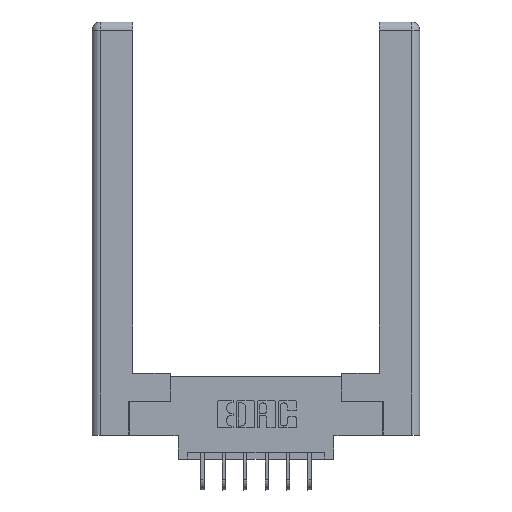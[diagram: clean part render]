
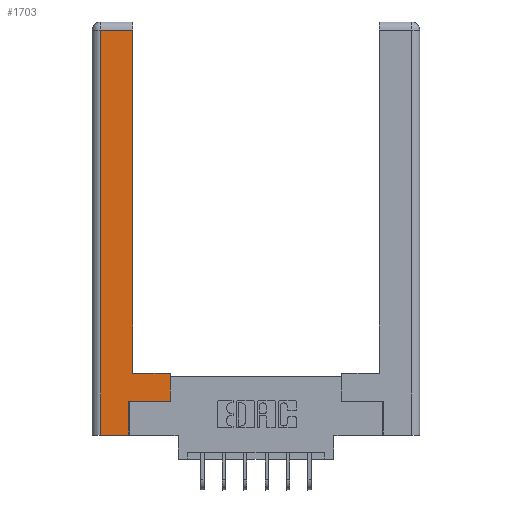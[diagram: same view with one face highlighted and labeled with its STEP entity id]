
A CAD part, top view. The second image highlights one B-rep face of the part: STEP entity #1703.
In plain terms, the highlighted planar face has unit normal (0, 0, 1).
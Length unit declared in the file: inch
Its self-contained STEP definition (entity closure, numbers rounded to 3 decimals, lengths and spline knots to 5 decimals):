
#116 = ORIENTED_EDGE ( 'NONE', *, *, #510, .T. ) ;
#121 = LINE ( 'NONE', #13574, #1933 ) ;
#510 = EDGE_CURVE ( 'NONE', #4263, #7107, #6602, .T. ) ;
#1077 = DIRECTION ( 'NONE',  ( -1., 0., 0. ) ) ;
#1200 = EDGE_CURVE ( 'NONE', #6168, #2631, #8794, .T. ) ;
#1439 = LINE ( 'NONE', #2901, #3430 ) ;
#1511 = EDGE_CURVE ( 'NONE', #7107, #2947, #5758, .T. ) ;
#1598 = CARTESIAN_POINT ( 'NONE',  ( 0.565, 0.245, 0. ) ) ;
#1703 = ADVANCED_FACE ( 'NONE', ( #5222 ), #13665, .F. ) ;
#1885 = CARTESIAN_POINT ( 'NONE',  ( 0., 0., 0. ) ) ;
#1933 = VECTOR ( 'NONE', #8411, 39.37008 ) ;
#2525 = CARTESIAN_POINT ( 'NONE',  ( 0.565, 0.45, 0. ) ) ;
#2631 = VERTEX_POINT ( 'NONE', #11453 ) ;
#2773 = LINE ( 'NONE', #13805, #7980 ) ;
#2901 = CARTESIAN_POINT ( 'NONE',  ( 0.565, 0.45, 0. ) ) ;
#2912 = VECTOR ( 'NONE', #9120, 39.37008 ) ;
#2947 = VERTEX_POINT ( 'NONE', #13669 ) ;
#3091 = DIRECTION ( 'NONE',  ( -1., 0., 0. ) ) ;
#3253 = CARTESIAN_POINT ( 'NONE',  ( 0.295, 0.45, 0. ) ) ;
#3430 = VECTOR ( 'NONE', #10761, 39.37008 ) ;
#3646 = CARTESIAN_POINT ( 'NONE',  ( 0.295, 2.94, 0. ) ) ;
#3906 = CARTESIAN_POINT ( 'NONE',  ( 0.265, 0.245, 0. ) ) ;
#4152 = CARTESIAN_POINT ( 'NONE',  ( 0.565, 0.245, 0. ) ) ;
#4263 = VERTEX_POINT ( 'NONE', #12890 ) ;
#4650 = CARTESIAN_POINT ( 'NONE',  ( 0.0615, 2.94, 0. ) ) ;
#4991 = CARTESIAN_POINT ( 'NONE',  ( 0.265, 0., 0. ) ) ;
#5222 = FACE_OUTER_BOUND ( 'NONE', #9736, .T. ) ;
#5223 = VERTEX_POINT ( 'NONE', #3646 ) ;
#5642 = ORIENTED_EDGE ( 'NONE', *, *, #6206, .T. ) ;
#5717 = ORIENTED_EDGE ( 'NONE', *, *, #13320, .T. ) ;
#5744 = EDGE_CURVE ( 'NONE', #2631, #5223, #121, .T. ) ;
#5758 = LINE ( 'NONE', #3906, #2912 ) ;
#5858 = EDGE_CURVE ( 'NONE', #5223, #12197, #2773, .T. ) ;
#6168 = VERTEX_POINT ( 'NONE', #2525 ) ;
#6206 = EDGE_CURVE ( 'NONE', #10298, #6168, #1439, .T. ) ;
#6342 = DIRECTION ( 'NONE',  ( -1., 0., 0. ) ) ;
#6602 = LINE ( 'NONE', #4991, #13525 ) ;
#7107 = VERTEX_POINT ( 'NONE', #13416 ) ;
#7304 = AXIS2_PLACEMENT_3D ( 'NONE', #1885, #9399, #6342 ) ;
#7393 = ORIENTED_EDGE ( 'NONE', *, *, #1511, .T. ) ;
#7461 = DIRECTION ( 'NONE',  ( 1., 0., 0. ) ) ;
#7565 = EDGE_CURVE ( 'NONE', #12197, #4263, #11890, .T. ) ;
#7685 = VECTOR ( 'NONE', #13307, 39.37008 ) ;
#7980 = VECTOR ( 'NONE', #3091, 39.37008 ) ;
#8226 = ORIENTED_EDGE ( 'NONE', *, *, #5744, .T. ) ;
#8255 = ORIENTED_EDGE ( 'NONE', *, *, #5858, .T. ) ;
#8410 = DIRECTION ( 'NONE',  ( 1., 0., 0. ) ) ;
#8411 = DIRECTION ( 'NONE',  ( 0., 1., 0. ) ) ;
#8794 = LINE ( 'NONE', #3253, #12163 ) ;
#9080 = CARTESIAN_POINT ( 'NONE',  ( 0.0615, 0., 0. ) ) ;
#9120 = DIRECTION ( 'NONE',  ( 0., 1., 0. ) ) ;
#9399 = DIRECTION ( 'NONE',  ( 0., 0., -1. ) ) ;
#9402 = VECTOR ( 'NONE', #8410, 39.37008 ) ;
#9736 = EDGE_LOOP ( 'NONE', ( #8226, #8255, #11293, #116, #7393, #5717, #5642, #11241 ) ) ;
#10298 = VERTEX_POINT ( 'NONE', #1598 ) ;
#10761 = DIRECTION ( 'NONE',  ( 0., 1., 0. ) ) ;
#11241 = ORIENTED_EDGE ( 'NONE', *, *, #1200, .T. ) ;
#11293 = ORIENTED_EDGE ( 'NONE', *, *, #7565, .T. ) ;
#11453 = CARTESIAN_POINT ( 'NONE',  ( 0.295, 0.45, 0. ) ) ;
#11890 = LINE ( 'NONE', #9080, #7685 ) ;
#12163 = VECTOR ( 'NONE', #1077, 39.37008 ) ;
#12197 = VERTEX_POINT ( 'NONE', #4650 ) ;
#12767 = LINE ( 'NONE', #4152, #9402 ) ;
#12890 = CARTESIAN_POINT ( 'NONE',  ( 0.0615, 0., 0. ) ) ;
#13307 = DIRECTION ( 'NONE',  ( 0., -1., 0. ) ) ;
#13320 = EDGE_CURVE ( 'NONE', #2947, #10298, #12767, .T. ) ;
#13416 = CARTESIAN_POINT ( 'NONE',  ( 0.265, 0., 0. ) ) ;
#13525 = VECTOR ( 'NONE', #7461, 39.37008 ) ;
#13574 = CARTESIAN_POINT ( 'NONE',  ( 0.295, 3., 0. ) ) ;
#13665 = PLANE ( 'NONE',  #7304 ) ;
#13669 = CARTESIAN_POINT ( 'NONE',  ( 0.265, 0.245, 0. ) ) ;
#13805 = CARTESIAN_POINT ( 'NONE',  ( 0.0615, 2.94, 0. ) ) ;
